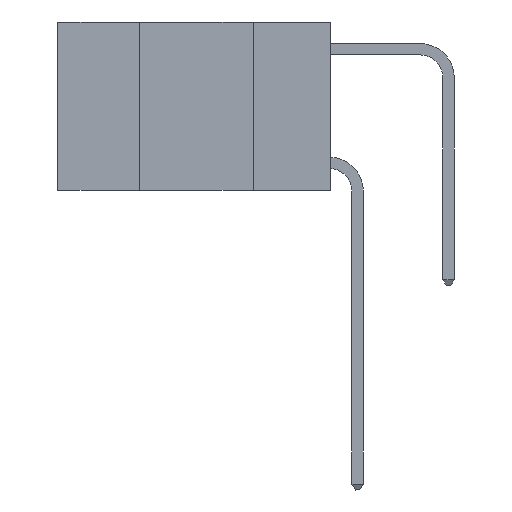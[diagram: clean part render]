
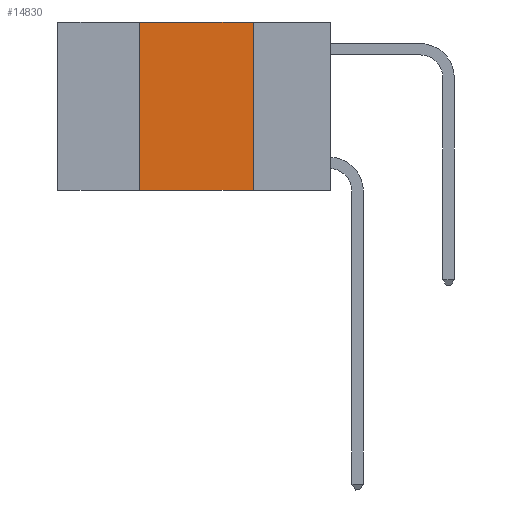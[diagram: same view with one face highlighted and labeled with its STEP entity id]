
A CAD part, left-side view. The second image highlights one B-rep face of the part: STEP entity #14830.
In plain terms, the highlighted planar face has unit normal (-1, 0, 0).
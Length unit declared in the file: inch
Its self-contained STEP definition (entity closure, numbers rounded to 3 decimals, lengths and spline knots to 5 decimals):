
#547 = DIRECTION ( 'NONE',  ( 0., -1., 0. ) ) ;
#779 = ORIENTED_EDGE ( 'NONE', *, *, #8165, .F. ) ;
#1063 = LINE ( 'NONE', #16530, #12104 ) ;
#1428 = VERTEX_POINT ( 'NONE', #3677 ) ;
#2035 = VERTEX_POINT ( 'NONE', #6485 ) ;
#2152 = PLANE ( 'NONE',  #7576 ) ;
#2520 = LINE ( 'NONE', #11041, #9422 ) ;
#2638 = DIRECTION ( 'NONE',  ( 0., -1., 0. ) ) ;
#3538 = FACE_OUTER_BOUND ( 'NONE', #7271, .T. ) ;
#3677 = CARTESIAN_POINT ( 'NONE',  ( 0., 0.17, 0. ) ) ;
#4388 = CARTESIAN_POINT ( 'NONE',  ( 0., 0.17, -0.37 ) ) ;
#4761 = EDGE_CURVE ( 'NONE', #2035, #13135, #4767, .T. ) ;
#4767 = LINE ( 'NONE', #10255, #13705 ) ;
#5214 = CARTESIAN_POINT ( 'NONE',  ( 0., 0.42, 0. ) ) ;
#5949 = EDGE_CURVE ( 'NONE', #1428, #13135, #2520, .T. ) ;
#6413 = ORIENTED_EDGE ( 'NONE', *, *, #4761, .T. ) ;
#6453 = CARTESIAN_POINT ( 'NONE',  ( 0., 0.42, 0. ) ) ;
#6485 = CARTESIAN_POINT ( 'NONE',  ( 0., 0.42, -0.37 ) ) ;
#7271 = EDGE_LOOP ( 'NONE', ( #9348, #779, #13516, #6413 ) ) ;
#7576 = AXIS2_PLACEMENT_3D ( 'NONE', #13263, #8954, #13176 ) ;
#8153 = DIRECTION ( 'NONE',  ( 0., 0., -1. ) ) ;
#8165 = EDGE_CURVE ( 'NONE', #8171, #1428, #1063, .T. ) ;
#8171 = VERTEX_POINT ( 'NONE', #5214 ) ;
#8218 = LINE ( 'NONE', #6453, #13014 ) ;
#8954 = DIRECTION ( 'NONE',  ( 1., 0., 0. ) ) ;
#9174 = EDGE_CURVE ( 'NONE', #2035, #8171, #8218, .T. ) ;
#9348 = ORIENTED_EDGE ( 'NONE', *, *, #5949, .F. ) ;
#9422 = VECTOR ( 'NONE', #8153, 39.37008 ) ;
#9470 = DIRECTION ( 'NONE',  ( 0., 0., 1. ) ) ;
#10255 = CARTESIAN_POINT ( 'NONE',  ( 0., 0.6, -0.37 ) ) ;
#11041 = CARTESIAN_POINT ( 'NONE',  ( 0., 0.17, 0. ) ) ;
#12104 = VECTOR ( 'NONE', #2638, 39.37008 ) ;
#13014 = VECTOR ( 'NONE', #9470, 39.37008 ) ;
#13135 = VERTEX_POINT ( 'NONE', #4388 ) ;
#13176 = DIRECTION ( 'NONE',  ( 0., 0., -1. ) ) ;
#13263 = CARTESIAN_POINT ( 'NONE',  ( 0., 0.6, 0. ) ) ;
#13516 = ORIENTED_EDGE ( 'NONE', *, *, #9174, .F. ) ;
#13705 = VECTOR ( 'NONE', #547, 39.37008 ) ;
#14830 = ADVANCED_FACE ( 'NONE', ( #3538 ), #2152, .F. ) ;
#16530 = CARTESIAN_POINT ( 'NONE',  ( 0., 0.6, 0. ) ) ;
